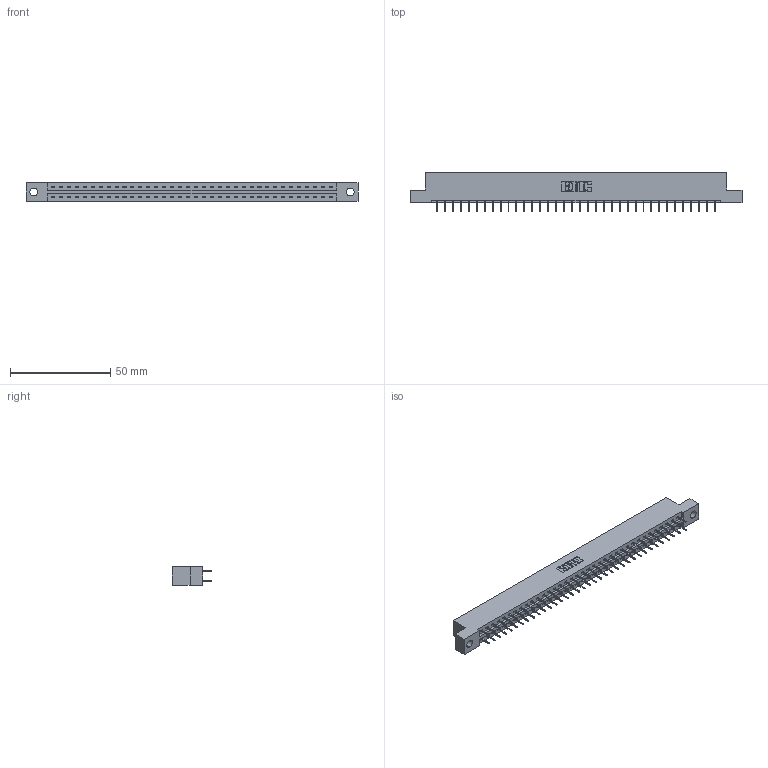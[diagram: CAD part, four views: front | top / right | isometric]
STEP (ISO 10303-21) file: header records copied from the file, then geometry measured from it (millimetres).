
FILE_DESCRIPTION (( 'STEP AP203' ), '1' );
FILE_NAME ('387-072-524-204.STEP', '2018-09-22T18:02:22', ( '' ), ( '' ), 'SwSTEP 2.0', 'SolidWorks 2016', '' );
FILE_SCHEMA (( 'CONFIG_CONTROL_DESIGN' ));
Length unit declared in the file: inch
Products named in the file (3): 337 Part_Flush Mounting Lugs - 0.156 Dia-TH; 345-292-001_345-293-124; 387-072-524-204
Assembly tree (73 placements, depth 2):
  387-072-524-204
    337 Part_Flush Mounting Lugs - 0.156 Dia-TH
    345-292-001_345-293-124  x72
Bounding box: 165.66 x 19.69 x 9.4 mm (x, y, z)
Volume: 17181.8 mm3; surface area: 18825.7 mm2
Topology: 73 solids, 73 shells, 4290 faces, 12191 edges, 7838 vertices
Faces by surface type: plane 3238, cylinder 1052
Entity records: 28765 total; most frequent: CARTESIAN_POINT 4850, ORIENTED_EDGE 4786, DIRECTION 4137, EDGE_CURVE 2393, LINE 2269, VECTOR 2269, VERTEX_POINT 1590, AXIS2_PLACEMENT_3D 934
